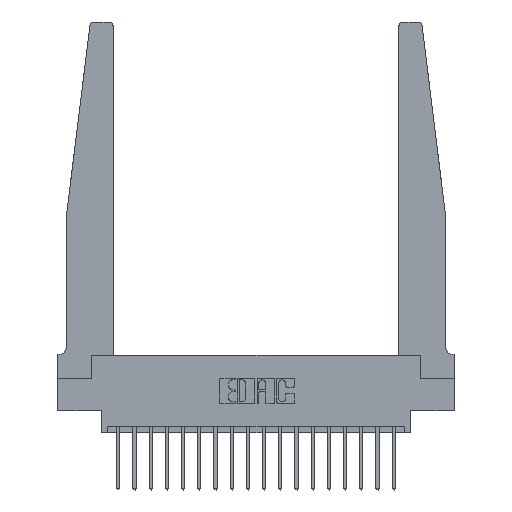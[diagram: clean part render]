
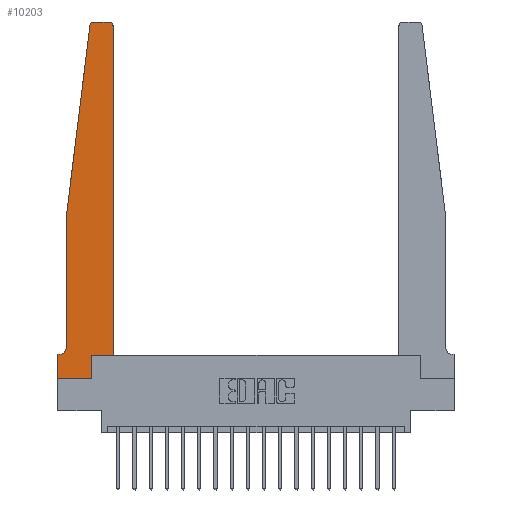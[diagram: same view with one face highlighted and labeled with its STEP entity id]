
A CAD part, top view. The second image highlights one B-rep face of the part: STEP entity #10203.
In plain terms, the highlighted planar face has unit normal (0, 0, 1).
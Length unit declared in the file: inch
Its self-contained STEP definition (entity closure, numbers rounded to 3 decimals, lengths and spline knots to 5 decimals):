
#430 = LINE ( 'NONE', #535, #5310 ) ;
#535 = CARTESIAN_POINT ( 'NONE',  ( 0., 0., 0.37 ) ) ;
#675 = FACE_OUTER_BOUND ( 'NONE', #3983, .T. ) ;
#928 = VECTOR ( 'NONE', #15646, 39.37008 ) ;
#975 = VERTEX_POINT ( 'NONE', #8431 ) ;
#1058 = CARTESIAN_POINT ( 'NONE',  ( 0.065, 1.25, 0.37 ) ) ;
#1152 = ORIENTED_EDGE ( 'NONE', *, *, #14969, .T. ) ;
#1164 = DIRECTION ( 'NONE',  ( -0.122, -0.992, 0. ) ) ;
#1543 = CARTESIAN_POINT ( 'NONE',  ( 0.425, 0.18, 0.37 ) ) ;
#2434 = VECTOR ( 'NONE', #13925, 39.37008 ) ;
#2441 = ORIENTED_EDGE ( 'NONE', *, *, #7698, .T. ) ;
#2495 = CARTESIAN_POINT ( 'NONE',  ( 0.015, 0.1875, 0.37 ) ) ;
#2923 = CARTESIAN_POINT ( 'NONE',  ( 0.24675, 2.72367, 0.37 ) ) ;
#3017 = VECTOR ( 'NONE', #10489, 39.37008 ) ;
#3087 = CARTESIAN_POINT ( 'NONE',  ( 0., 0.1875, 0.37 ) ) ;
#3694 = CARTESIAN_POINT ( 'NONE',  ( 0.27653, 2.75, 0.37 ) ) ;
#3983 = EDGE_LOOP ( 'NONE', ( #16275, #1152, #16945, #8240, #4288, #2441, #7439, #15647, #5790, #6096, #4040, #14472 ) ) ;
#4040 = ORIENTED_EDGE ( 'NONE', *, *, #18083, .T. ) ;
#4273 = LINE ( 'NONE', #10558, #5421 ) ;
#4288 = ORIENTED_EDGE ( 'NONE', *, *, #17722, .T. ) ;
#4429 = VECTOR ( 'NONE', #1164, 39.37008 ) ;
#4462 = LINE ( 'NONE', #16877, #19182 ) ;
#5310 = VECTOR ( 'NONE', #16367, 39.37008 ) ;
#5421 = VECTOR ( 'NONE', #11896, 39.37008 ) ;
#5607 = CARTESIAN_POINT ( 'NONE',  ( 0.065, 1.25, 0.37 ) ) ;
#5790 = ORIENTED_EDGE ( 'NONE', *, *, #13824, .T. ) ;
#5911 = LINE ( 'NONE', #10658, #9755 ) ;
#6084 = EDGE_CURVE ( 'NONE', #17079, #6952, #5911, .T. ) ;
#6096 = ORIENTED_EDGE ( 'NONE', *, *, #6084, .T. ) ;
#6412 = CIRCLE ( 'NONE', #7062, 0.03 ) ;
#6752 = VERTEX_POINT ( 'NONE', #11554 ) ;
#6952 = VERTEX_POINT ( 'NONE', #1543 ) ;
#6968 = PLANE ( 'NONE',  #12370 ) ;
#7059 = VERTEX_POINT ( 'NONE', #3087 ) ;
#7062 = AXIS2_PLACEMENT_3D ( 'NONE', #11028, #7928, #12659 ) ;
#7182 = VERTEX_POINT ( 'NONE', #5607 ) ;
#7392 = VERTEX_POINT ( 'NONE', #8186 ) ;
#7439 = ORIENTED_EDGE ( 'NONE', *, *, #13295, .T. ) ;
#7698 = EDGE_CURVE ( 'NONE', #10540, #7059, #9583, .T. ) ;
#7928 = DIRECTION ( 'NONE',  ( 0., 0., 1. ) ) ;
#8006 = CARTESIAN_POINT ( 'NONE',  ( 0.015, 0.2375, 0.37 ) ) ;
#8186 = CARTESIAN_POINT ( 'NONE',  ( 0., 0., 0.37 ) ) ;
#8213 = DIRECTION ( 'NONE',  ( 0., 0., 1. ) ) ;
#8240 = ORIENTED_EDGE ( 'NONE', *, *, #18634, .T. ) ;
#8418 = CARTESIAN_POINT ( 'NONE',  ( 0.25, 2.75, 0.37 ) ) ;
#8431 = CARTESIAN_POINT ( 'NONE',  ( 0.425, 2.72, 0.37 ) ) ;
#8647 = DIRECTION ( 'NONE',  ( 1., 0., 0. ) ) ;
#8784 = CARTESIAN_POINT ( 'NONE',  ( 0.2605, 0.18, 0.37 ) ) ;
#8981 = CARTESIAN_POINT ( 'NONE',  ( 0.065, 1.25, 0.37 ) ) ;
#9583 = LINE ( 'NONE', #11149, #928 ) ;
#9755 = VECTOR ( 'NONE', #11890, 39.37008 ) ;
#9830 = LINE ( 'NONE', #1058, #4429 ) ;
#10167 = DIRECTION ( 'NONE',  ( -1., 0., 0. ) ) ;
#10203 = ADVANCED_FACE ( 'NONE', ( #675 ), #6968, .T. ) ;
#10489 = DIRECTION ( 'NONE',  ( 0., 1., 0. ) ) ;
#10540 = VERTEX_POINT ( 'NONE', #2495 ) ;
#10558 = CARTESIAN_POINT ( 'NONE',  ( 0.425, 0.18, 0.37 ) ) ;
#10622 = VERTEX_POINT ( 'NONE', #14840 ) ;
#10658 = CARTESIAN_POINT ( 'NONE',  ( 0.425, 0.18, 0.37 ) ) ;
#11028 = CARTESIAN_POINT ( 'NONE',  ( 0.395, 2.72, 0.37 ) ) ;
#11149 = CARTESIAN_POINT ( 'NONE',  ( 0.065, 0.1875, 0.37 ) ) ;
#11396 = EDGE_CURVE ( 'NONE', #10622, #15929, #11605, .T. ) ;
#11554 = CARTESIAN_POINT ( 'NONE',  ( 0.065, 0.2375, 0.37 ) ) ;
#11563 = EDGE_CURVE ( 'NONE', #18672, #7182, #9830, .T. ) ;
#11605 = LINE ( 'NONE', #8418, #20077 ) ;
#11890 = DIRECTION ( 'NONE',  ( 1., 0., 0. ) ) ;
#11896 = DIRECTION ( 'NONE',  ( 0., 1., 0. ) ) ;
#12214 = VERTEX_POINT ( 'NONE', #14116 ) ;
#12370 = AXIS2_PLACEMENT_3D ( 'NONE', #13245, #8213, #17952 ) ;
#12579 = DIRECTION ( 'NONE',  ( 1., 0., 0. ) ) ;
#12659 = DIRECTION ( 'NONE',  ( 1., 0., 0. ) ) ;
#12982 = AXIS2_PLACEMENT_3D ( 'NONE', #8006, #18892, #16928 ) ;
#13182 = DIRECTION ( 'NONE',  ( 0., 0., 1. ) ) ;
#13245 = CARTESIAN_POINT ( 'NONE',  ( 0., 0.1875, 0.37 ) ) ;
#13295 = EDGE_CURVE ( 'NONE', #7059, #7392, #430, .T. ) ;
#13824 = EDGE_CURVE ( 'NONE', #12214, #17079, #18085, .T. ) ;
#13925 = DIRECTION ( 'NONE',  ( 0., -1., 0. ) ) ;
#14116 = CARTESIAN_POINT ( 'NONE',  ( 0.2605, 0., 0.37 ) ) ;
#14472 = ORIENTED_EDGE ( 'NONE', *, *, #17262, .T. ) ;
#14840 = CARTESIAN_POINT ( 'NONE',  ( 0.395, 2.75, 0.37 ) ) ;
#14874 = CIRCLE ( 'NONE', #16181, 0.03 ) ;
#14968 = CIRCLE ( 'NONE', #12982, 0.05 ) ;
#14969 = EDGE_CURVE ( 'NONE', #15929, #18672, #14874, .T. ) ;
#15456 = LINE ( 'NONE', #8981, #2434 ) ;
#15646 = DIRECTION ( 'NONE',  ( -1., 0., 0. ) ) ;
#15647 = ORIENTED_EDGE ( 'NONE', *, *, #18653, .T. ) ;
#15878 = CARTESIAN_POINT ( 'NONE',  ( 0.27653, 2.72, 0.37 ) ) ;
#15929 = VERTEX_POINT ( 'NONE', #3694 ) ;
#16181 = AXIS2_PLACEMENT_3D ( 'NONE', #15878, #13182, #8647 ) ;
#16275 = ORIENTED_EDGE ( 'NONE', *, *, #11396, .T. ) ;
#16367 = DIRECTION ( 'NONE',  ( 0., -1., 0. ) ) ;
#16877 = CARTESIAN_POINT ( 'NONE',  ( 0., 0., 0.37 ) ) ;
#16928 = DIRECTION ( 'NONE',  ( -1., 0., 0. ) ) ;
#16945 = ORIENTED_EDGE ( 'NONE', *, *, #11563, .T. ) ;
#17079 = VERTEX_POINT ( 'NONE', #8784 ) ;
#17262 = EDGE_CURVE ( 'NONE', #975, #10622, #6412, .T. ) ;
#17722 = EDGE_CURVE ( 'NONE', #6752, #10540, #14968, .T. ) ;
#17952 = DIRECTION ( 'NONE',  ( 1., 0., 0. ) ) ;
#18083 = EDGE_CURVE ( 'NONE', #6952, #975, #4273, .T. ) ;
#18085 = LINE ( 'NONE', #18285, #3017 ) ;
#18285 = CARTESIAN_POINT ( 'NONE',  ( 0.2605, 0.18, 0.37 ) ) ;
#18634 = EDGE_CURVE ( 'NONE', #7182, #6752, #15456, .T. ) ;
#18653 = EDGE_CURVE ( 'NONE', #7392, #12214, #4462, .T. ) ;
#18672 = VERTEX_POINT ( 'NONE', #2923 ) ;
#18892 = DIRECTION ( 'NONE',  ( 0., 0., -1. ) ) ;
#19182 = VECTOR ( 'NONE', #12579, 39.37008 ) ;
#20077 = VECTOR ( 'NONE', #10167, 39.37008 ) ;
